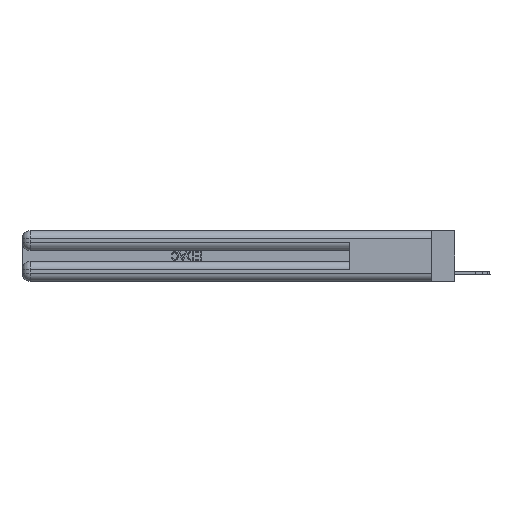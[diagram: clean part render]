
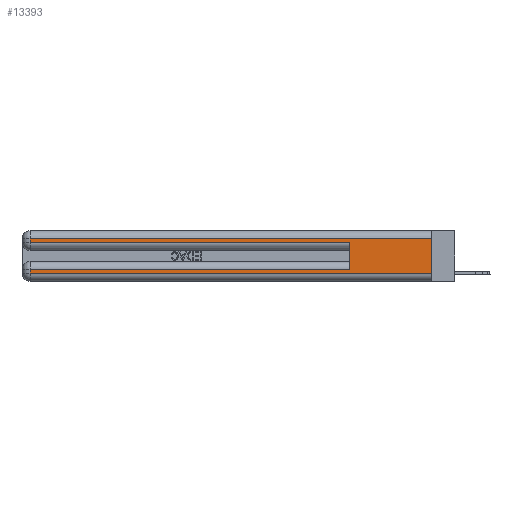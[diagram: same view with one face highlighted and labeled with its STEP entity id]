
A CAD part, left-side view. The second image highlights one B-rep face of the part: STEP entity #13393.
In plain terms, the highlighted planar face has unit normal (-1, 0, 0).
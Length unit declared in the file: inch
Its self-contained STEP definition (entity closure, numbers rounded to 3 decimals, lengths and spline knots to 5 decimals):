
#203 = ORIENTED_EDGE ( 'NONE', *, *, #11616, .T. ) ;
#453 = CARTESIAN_POINT ( 'NONE',  ( 0., 2.94, 0.31 ) ) ;
#593 = VERTEX_POINT ( 'NONE', #1705 ) ;
#793 = AXIS2_PLACEMENT_3D ( 'NONE', #22054, #20843, #13653 ) ;
#1705 = CARTESIAN_POINT ( 'NONE',  ( 0., 0.6, 0.085 ) ) ;
#2097 = LINE ( 'NONE', #22893, #16011 ) ;
#2791 = LINE ( 'NONE', #5149, #10301 ) ;
#3501 = ORIENTED_EDGE ( 'NONE', *, *, #7066, .T. ) ;
#4448 = EDGE_CURVE ( 'NONE', #14145, #11819, #2097, .T. ) ;
#4477 = DIRECTION ( 'NONE',  ( 0., -1., 0. ) ) ;
#4544 = DIRECTION ( 'NONE',  ( 0., 1., 0. ) ) ;
#5104 = EDGE_CURVE ( 'NONE', #593, #11819, #2791, .T. ) ;
#5149 = CARTESIAN_POINT ( 'NONE',  ( 0., 0.6, 0.145 ) ) ;
#5916 = VERTEX_POINT ( 'NONE', #11558 ) ;
#5972 = LINE ( 'NONE', #10856, #7232 ) ;
#6526 = CARTESIAN_POINT ( 'NONE',  ( 0., 0., 0.06 ) ) ;
#7066 = EDGE_CURVE ( 'NONE', #24816, #18558, #12705, .T. ) ;
#7232 = VECTOR ( 'NONE', #19849, 39.37008 ) ;
#8580 = DIRECTION ( 'NONE',  ( 0., 0., -1. ) ) ;
#9016 = CARTESIAN_POINT ( 'NONE',  ( 0., 2.94, 0.37 ) ) ;
#9093 = CARTESIAN_POINT ( 'NONE',  ( 0., 0., 0.37 ) ) ;
#9342 = VECTOR ( 'NONE', #8580, 39.37008 ) ;
#9465 = ORIENTED_EDGE ( 'NONE', *, *, #4448, .T. ) ;
#9822 = ORIENTED_EDGE ( 'NONE', *, *, #5104, .F. ) ;
#10301 = VECTOR ( 'NONE', #10436, 39.37008 ) ;
#10329 = DIRECTION ( 'NONE',  ( 0., 1., 0. ) ) ;
#10436 = DIRECTION ( 'NONE',  ( 0., 0., 1. ) ) ;
#10856 = CARTESIAN_POINT ( 'NONE',  ( 0., 2.94, 0.37 ) ) ;
#10992 = LINE ( 'NONE', #9093, #22171 ) ;
#11558 = CARTESIAN_POINT ( 'NONE',  ( 0., 0., 0.06 ) ) ;
#11616 = EDGE_CURVE ( 'NONE', #593, #26027, #18092, .T. ) ;
#11819 = VERTEX_POINT ( 'NONE', #19835 ) ;
#12271 = ORIENTED_EDGE ( 'NONE', *, *, #27437, .T. ) ;
#12386 = ORIENTED_EDGE ( 'NONE', *, *, #23312, .F. ) ;
#12705 = LINE ( 'NONE', #19046, #14795 ) ;
#13374 = CARTESIAN_POINT ( 'NONE',  ( 0., 0., 0.31 ) ) ;
#13393 = ADVANCED_FACE ( 'NONE', ( #26510 ), #24306, .F. ) ;
#13653 = DIRECTION ( 'NONE',  ( 0., 0., -1. ) ) ;
#13994 = VERTEX_POINT ( 'NONE', #20445 ) ;
#14145 = VERTEX_POINT ( 'NONE', #21588 ) ;
#14795 = VECTOR ( 'NONE', #10329, 39.37008 ) ;
#15667 = VECTOR ( 'NONE', #4544, 39.37008 ) ;
#16011 = VECTOR ( 'NONE', #18016, 39.37008 ) ;
#17899 = DIRECTION ( 'NONE',  ( 0., 0., -1. ) ) ;
#18016 = DIRECTION ( 'NONE',  ( 0., -1., 0. ) ) ;
#18092 = LINE ( 'NONE', #24894, #15667 ) ;
#18558 = VERTEX_POINT ( 'NONE', #453 ) ;
#19046 = CARTESIAN_POINT ( 'NONE',  ( 0., 0., 0.31 ) ) ;
#19835 = CARTESIAN_POINT ( 'NONE',  ( 0., 0.6, 0.285 ) ) ;
#19849 = DIRECTION ( 'NONE',  ( 0., 0., -1. ) ) ;
#20445 = CARTESIAN_POINT ( 'NONE',  ( 0., 2.94, 0.06 ) ) ;
#20843 = DIRECTION ( 'NONE',  ( 1., 0., 0. ) ) ;
#20964 = EDGE_CURVE ( 'NONE', #18558, #14145, #5972, .T. ) ;
#21588 = CARTESIAN_POINT ( 'NONE',  ( 0., 2.94, 0.285 ) ) ;
#22054 = CARTESIAN_POINT ( 'NONE',  ( 0., 0., 0.37 ) ) ;
#22171 = VECTOR ( 'NONE', #17899, 39.37008 ) ;
#22893 = CARTESIAN_POINT ( 'NONE',  ( 0., 0., 0.285 ) ) ;
#23217 = VECTOR ( 'NONE', #4477, 39.37008 ) ;
#23312 = EDGE_CURVE ( 'NONE', #24816, #5916, #10992, .T. ) ;
#24080 = CARTESIAN_POINT ( 'NONE',  ( 0., 2.94, 0.085 ) ) ;
#24306 = PLANE ( 'NONE',  #793 ) ;
#24816 = VERTEX_POINT ( 'NONE', #13374 ) ;
#24894 = CARTESIAN_POINT ( 'NONE',  ( 0., 0., 0.085 ) ) ;
#25775 = ORIENTED_EDGE ( 'NONE', *, *, #20964, .T. ) ;
#26027 = VERTEX_POINT ( 'NONE', #24080 ) ;
#26239 = EDGE_LOOP ( 'NONE', ( #12386, #3501, #25775, #9465, #9822, #203, #12271, #28474 ) ) ;
#26510 = FACE_OUTER_BOUND ( 'NONE', #26239, .T. ) ;
#26599 = LINE ( 'NONE', #9016, #9342 ) ;
#26911 = LINE ( 'NONE', #6526, #23217 ) ;
#27437 = EDGE_CURVE ( 'NONE', #26027, #13994, #26599, .T. ) ;
#28339 = EDGE_CURVE ( 'NONE', #13994, #5916, #26911, .T. ) ;
#28474 = ORIENTED_EDGE ( 'NONE', *, *, #28339, .T. ) ;
